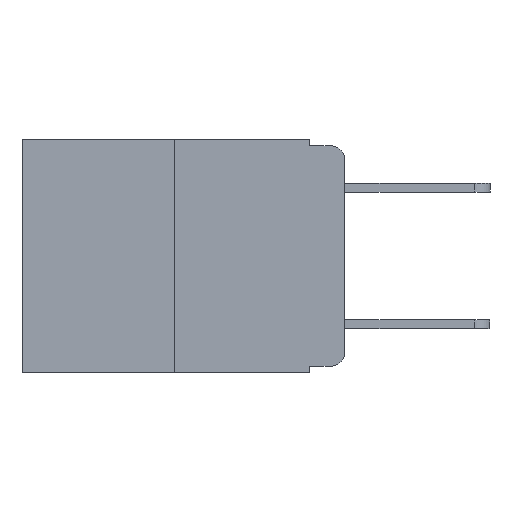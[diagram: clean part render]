
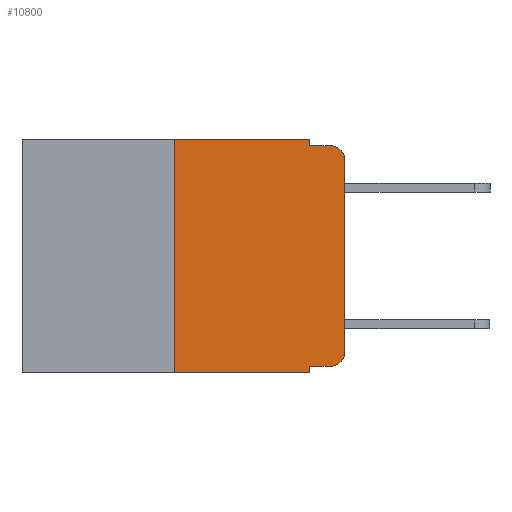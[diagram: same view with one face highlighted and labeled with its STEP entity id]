
A CAD part, left-side view. The second image highlights one B-rep face of the part: STEP entity #10800.
In plain terms, the highlighted planar face has unit normal (-1, 0, 0).
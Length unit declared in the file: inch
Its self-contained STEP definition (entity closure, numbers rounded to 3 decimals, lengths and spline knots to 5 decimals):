
#306 = EDGE_CURVE ( 'NONE', #11368, #4239, #9098, .T. ) ;
#339 = CARTESIAN_POINT ( 'NONE',  ( 0., 0., -0.313 ) ) ;
#415 = ORIENTED_EDGE ( 'NONE', *, *, #1627, .F. ) ;
#692 = AXIS2_PLACEMENT_3D ( 'NONE', #7243, #1307, #8201 ) ;
#743 = ORIENTED_EDGE ( 'NONE', *, *, #2374, .F. ) ;
#1282 = EDGE_CURVE ( 'NONE', #7723, #4239, #7491, .T. ) ;
#1307 = DIRECTION ( 'NONE',  ( -1., 0., 0. ) ) ;
#1342 = EDGE_CURVE ( 'NONE', #7723, #11351, #6545, .T. ) ;
#1361 = EDGE_CURVE ( 'NONE', #11351, #6499, #5616, .T. ) ;
#1427 = EDGE_CURVE ( 'NONE', #6499, #7949, #2392, .T. ) ;
#1452 = EDGE_CURVE ( 'NONE', #7949, #2546, #7333, .T. ) ;
#1627 = EDGE_CURVE ( 'NONE', #5804, #2546, #2706, .T. ) ;
#1719 = ORIENTED_EDGE ( 'NONE', *, *, #306, .T. ) ;
#1989 = CARTESIAN_POINT ( 'NONE',  ( 0., 0.02, -0.01 ) ) ;
#2035 = ORIENTED_EDGE ( 'NONE', *, *, #1342, .T. ) ;
#2062 = DIRECTION ( 'NONE',  ( 0., -1., 0. ) ) ;
#2068 = LINE ( 'NONE', #4037, #4657 ) ;
#2141 = LINE ( 'NONE', #2373, #7109 ) ;
#2222 = VERTEX_POINT ( 'NONE', #8382 ) ;
#2373 = CARTESIAN_POINT ( 'NONE',  ( 0., 0.25, 0. ) ) ;
#2374 = EDGE_CURVE ( 'NONE', #11300, #5804, #7415, .T. ) ;
#2392 = LINE ( 'NONE', #7162, #9762 ) ;
#2544 = CARTESIAN_POINT ( 'NONE',  ( 0., 0.051, 0. ) ) ;
#2546 = VERTEX_POINT ( 'NONE', #1989 ) ;
#2706 = LINE ( 'NONE', #7492, #7645 ) ;
#2761 = EDGE_CURVE ( 'NONE', #11368, #2222, #2141, .T. ) ;
#3327 = CARTESIAN_POINT ( 'NONE',  ( 0., 0.473, -0.343 ) ) ;
#3420 = ORIENTED_EDGE ( 'NONE', *, *, #5781, .F. ) ;
#3625 = CARTESIAN_POINT ( 'NONE',  ( 0., 0.02, -0.333 ) ) ;
#4037 = CARTESIAN_POINT ( 'NONE',  ( 0., 0.473, 0. ) ) ;
#4076 = CARTESIAN_POINT ( 'NONE',  ( 0., 0.02, -0.313 ) ) ;
#4239 = VERTEX_POINT ( 'NONE', #9689 ) ;
#4316 = ORIENTED_EDGE ( 'NONE', *, *, #1282, .F. ) ;
#4657 = VECTOR ( 'NONE', #2062, 39.37008 ) ;
#4756 = DIRECTION ( 'NONE',  ( 1., 0., 0. ) ) ;
#4836 = DIRECTION ( 'NONE',  ( 0., 0., -1. ) ) ;
#5056 = DIRECTION ( 'NONE',  ( 0., 0., -1. ) ) ;
#5616 = CIRCLE ( 'NONE', #8234, 0.02 ) ;
#5781 = EDGE_CURVE ( 'NONE', #2222, #11300, #2068, .T. ) ;
#5804 = VERTEX_POINT ( 'NONE', #8885 ) ;
#5891 = CARTESIAN_POINT ( 'NONE',  ( 0., 0.051, -0.333 ) ) ;
#5973 = DIRECTION ( 'NONE',  ( 0., -1., 0. ) ) ;
#6230 = DIRECTION ( 'NONE',  ( 0., -1., 0. ) ) ;
#6239 = VECTOR ( 'NONE', #5973, 39.37008 ) ;
#6499 = VERTEX_POINT ( 'NONE', #339 ) ;
#6545 = LINE ( 'NONE', #9727, #6239 ) ;
#6582 = CARTESIAN_POINT ( 'NONE',  ( 0., 0.25, -0.343 ) ) ;
#7109 = VECTOR ( 'NONE', #9153, 39.37008 ) ;
#7162 = CARTESIAN_POINT ( 'NONE',  ( 0., 0., 0. ) ) ;
#7243 = CARTESIAN_POINT ( 'NONE',  ( 0., 0.02, -0.03 ) ) ;
#7333 = CIRCLE ( 'NONE', #692, 0.02 ) ;
#7415 = LINE ( 'NONE', #10355, #9009 ) ;
#7491 = LINE ( 'NONE', #11392, #9346 ) ;
#7492 = CARTESIAN_POINT ( 'NONE',  ( 0., 0.051, -0.01 ) ) ;
#7639 = DIRECTION ( 'NONE',  ( 0., 0., -1. ) ) ;
#7645 = VECTOR ( 'NONE', #9327, 39.37008 ) ;
#7679 = PLANE ( 'NONE',  #11019 ) ;
#7723 = VERTEX_POINT ( 'NONE', #5891 ) ;
#7949 = VERTEX_POINT ( 'NONE', #9103 ) ;
#8028 = ORIENTED_EDGE ( 'NONE', *, *, #1452, .T. ) ;
#8201 = DIRECTION ( 'NONE',  ( 0., 0., -1. ) ) ;
#8234 = AXIS2_PLACEMENT_3D ( 'NONE', #4076, #10674, #5056 ) ;
#8382 = CARTESIAN_POINT ( 'NONE',  ( 0., 0.25, 0. ) ) ;
#8461 = FACE_OUTER_BOUND ( 'NONE', #10402, .T. ) ;
#8885 = CARTESIAN_POINT ( 'NONE',  ( 0., 0.051, -0.01 ) ) ;
#9009 = VECTOR ( 'NONE', #7639, 39.37008 ) ;
#9098 = LINE ( 'NONE', #3327, #11161 ) ;
#9103 = CARTESIAN_POINT ( 'NONE',  ( 0., 0., -0.03 ) ) ;
#9153 = DIRECTION ( 'NONE',  ( 0., 0., 1. ) ) ;
#9327 = DIRECTION ( 'NONE',  ( 0., -1., 0. ) ) ;
#9346 = VECTOR ( 'NONE', #4836, 39.37008 ) ;
#9549 = CARTESIAN_POINT ( 'NONE',  ( 0., 0.473, 0. ) ) ;
#9689 = CARTESIAN_POINT ( 'NONE',  ( 0., 0.051, -0.343 ) ) ;
#9721 = ORIENTED_EDGE ( 'NONE', *, *, #1361, .T. ) ;
#9727 = CARTESIAN_POINT ( 'NONE',  ( 0., 0.051, -0.333 ) ) ;
#9762 = VECTOR ( 'NONE', #11642, 39.37008 ) ;
#10355 = CARTESIAN_POINT ( 'NONE',  ( 0., 0.051, 0. ) ) ;
#10402 = EDGE_LOOP ( 'NONE', ( #11893, #8028, #415, #743, #3420, #10945, #1719, #4316, #2035, #9721 ) ) ;
#10674 = DIRECTION ( 'NONE',  ( -1., 0., 0. ) ) ;
#10800 = ADVANCED_FACE ( 'NONE', ( #8461 ), #7679, .F. ) ;
#10945 = ORIENTED_EDGE ( 'NONE', *, *, #2761, .F. ) ;
#11019 = AXIS2_PLACEMENT_3D ( 'NONE', #9549, #4756, #11326 ) ;
#11161 = VECTOR ( 'NONE', #6230, 39.37008 ) ;
#11300 = VERTEX_POINT ( 'NONE', #2544 ) ;
#11326 = DIRECTION ( 'NONE',  ( 0., 0., -1. ) ) ;
#11351 = VERTEX_POINT ( 'NONE', #3625 ) ;
#11368 = VERTEX_POINT ( 'NONE', #6582 ) ;
#11392 = CARTESIAN_POINT ( 'NONE',  ( 0., 0.051, 0. ) ) ;
#11642 = DIRECTION ( 'NONE',  ( 0., 0., 1. ) ) ;
#11893 = ORIENTED_EDGE ( 'NONE', *, *, #1427, .T. ) ;
